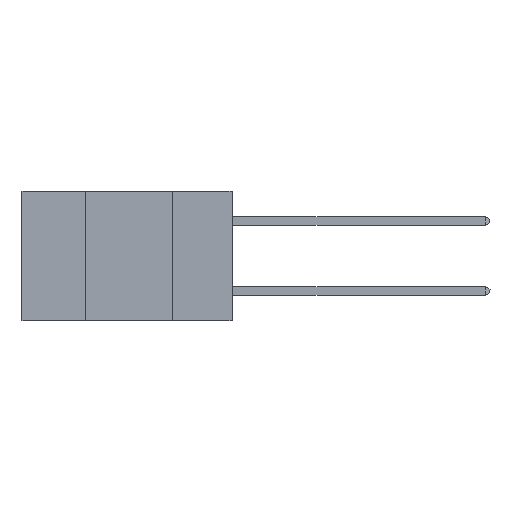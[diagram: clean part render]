
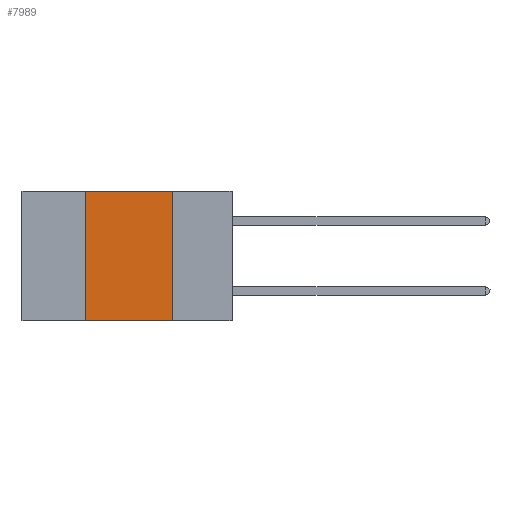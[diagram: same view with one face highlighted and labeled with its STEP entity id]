
A CAD part, left-side view. The second image highlights one B-rep face of the part: STEP entity #7989.
In plain terms, the highlighted planar face has unit normal (-1, 0, 0).
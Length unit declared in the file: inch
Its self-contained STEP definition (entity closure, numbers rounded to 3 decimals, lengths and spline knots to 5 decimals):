
#887 = DIRECTION ( 'NONE',  ( 1., 0., 0. ) ) ;
#1079 = FACE_OUTER_BOUND ( 'NONE', #6138, .T. ) ;
#1228 = CARTESIAN_POINT ( 'NONE',  ( 0., 0.42, -0.37 ) ) ;
#1522 = DIRECTION ( 'NONE',  ( 0., -1., 0. ) ) ;
#1552 = EDGE_CURVE ( 'NONE', #9650, #6463, #8447, .T. ) ;
#2002 = ORIENTED_EDGE ( 'NONE', *, *, #1552, .F. ) ;
#2070 = DIRECTION ( 'NONE',  ( 0., 0., 1. ) ) ;
#2150 = ORIENTED_EDGE ( 'NONE', *, *, #5966, .F. ) ;
#2497 = AXIS2_PLACEMENT_3D ( 'NONE', #8112, #887, #10355 ) ;
#3444 = CARTESIAN_POINT ( 'NONE',  ( 0., 0.17, 0. ) ) ;
#3548 = CARTESIAN_POINT ( 'NONE',  ( 0., 0.42, 0. ) ) ;
#4414 = EDGE_CURVE ( 'NONE', #6463, #9504, #6663, .T. ) ;
#4429 = CARTESIAN_POINT ( 'NONE',  ( 0., 0.17, -0.37 ) ) ;
#4575 = CARTESIAN_POINT ( 'NONE',  ( 0., 0.42, 0. ) ) ;
#4745 = DIRECTION ( 'NONE',  ( 0., 0., -1. ) ) ;
#4989 = VECTOR ( 'NONE', #1522, 39.37008 ) ;
#5966 = EDGE_CURVE ( 'NONE', #9504, #8875, #10233, .T. ) ;
#6138 = EDGE_LOOP ( 'NONE', ( #2150, #8041, #2002, #8917 ) ) ;
#6290 = VECTOR ( 'NONE', #2070, 39.37008 ) ;
#6363 = LINE ( 'NONE', #9423, #4989 ) ;
#6463 = VERTEX_POINT ( 'NONE', #4575 ) ;
#6663 = LINE ( 'NONE', #10001, #9159 ) ;
#7989 = ADVANCED_FACE ( 'NONE', ( #1079 ), #8770, .F. ) ;
#8041 = ORIENTED_EDGE ( 'NONE', *, *, #4414, .F. ) ;
#8112 = CARTESIAN_POINT ( 'NONE',  ( 0., 0.6, 0. ) ) ;
#8447 = LINE ( 'NONE', #3548, #6290 ) ;
#8770 = PLANE ( 'NONE',  #2497 ) ;
#8875 = VERTEX_POINT ( 'NONE', #4429 ) ;
#8917 = ORIENTED_EDGE ( 'NONE', *, *, #9143, .T. ) ;
#9105 = DIRECTION ( 'NONE',  ( 0., -1., 0. ) ) ;
#9143 = EDGE_CURVE ( 'NONE', #9650, #8875, #6363, .T. ) ;
#9159 = VECTOR ( 'NONE', #9105, 39.37008 ) ;
#9423 = CARTESIAN_POINT ( 'NONE',  ( 0., 0.6, -0.37 ) ) ;
#9450 = CARTESIAN_POINT ( 'NONE',  ( 0., 0.17, 0. ) ) ;
#9504 = VERTEX_POINT ( 'NONE', #3444 ) ;
#9650 = VERTEX_POINT ( 'NONE', #1228 ) ;
#10001 = CARTESIAN_POINT ( 'NONE',  ( 0., 0.6, 0. ) ) ;
#10123 = VECTOR ( 'NONE', #4745, 39.37008 ) ;
#10233 = LINE ( 'NONE', #9450, #10123 ) ;
#10355 = DIRECTION ( 'NONE',  ( 0., 0., -1. ) ) ;
